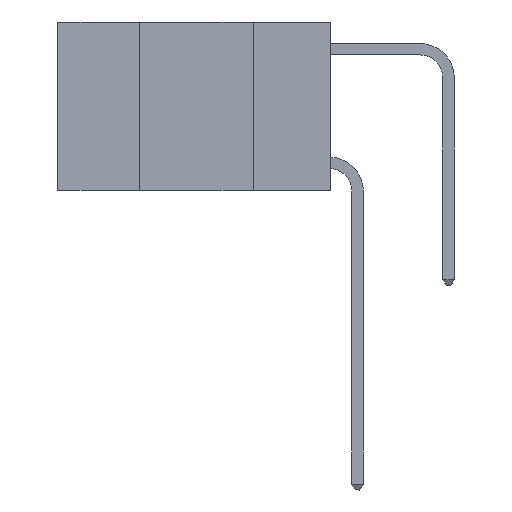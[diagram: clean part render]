
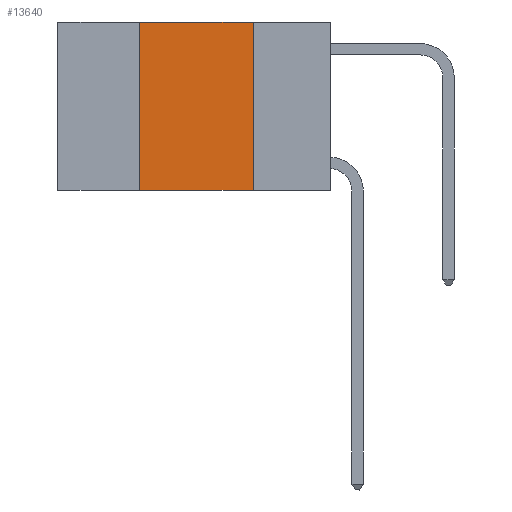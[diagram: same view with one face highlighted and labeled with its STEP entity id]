
A CAD part, left-side view. The second image highlights one B-rep face of the part: STEP entity #13640.
In plain terms, the highlighted planar face has unit normal (-1, 0, 0).
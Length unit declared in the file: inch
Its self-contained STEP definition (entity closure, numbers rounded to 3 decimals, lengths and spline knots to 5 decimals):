
#929 = VERTEX_POINT ( 'NONE', #13908 ) ;
#985 = ORIENTED_EDGE ( 'NONE', *, *, #4990, .F. ) ;
#1017 = VECTOR ( 'NONE', #14327, 39.37008 ) ;
#1131 = DIRECTION ( 'NONE',  ( 1., 0., 0. ) ) ;
#2269 = CARTESIAN_POINT ( 'NONE',  ( 0., 0.42, 0. ) ) ;
#4297 = EDGE_CURVE ( 'NONE', #929, #8619, #11769, .T. ) ;
#4489 = CARTESIAN_POINT ( 'NONE',  ( 0., 0.42, -0.37 ) ) ;
#4491 = CARTESIAN_POINT ( 'NONE',  ( 0., 0.17, -0.37 ) ) ;
#4765 = CARTESIAN_POINT ( 'NONE',  ( 0., 0.6, 0. ) ) ;
#4874 = VECTOR ( 'NONE', #16070, 39.37008 ) ;
#4990 = EDGE_CURVE ( 'NONE', #9619, #929, #16143, .T. ) ;
#5098 = ORIENTED_EDGE ( 'NONE', *, *, #14146, .F. ) ;
#5395 = VECTOR ( 'NONE', #12806, 39.37008 ) ;
#5797 = VECTOR ( 'NONE', #14953, 39.37008 ) ;
#6696 = FACE_OUTER_BOUND ( 'NONE', #9792, .T. ) ;
#8085 = CARTESIAN_POINT ( 'NONE',  ( 0., 0.42, 0. ) ) ;
#8619 = VERTEX_POINT ( 'NONE', #4491 ) ;
#8660 = CARTESIAN_POINT ( 'NONE',  ( 0., 0.17, 0. ) ) ;
#8819 = ORIENTED_EDGE ( 'NONE', *, *, #12000, .T. ) ;
#9490 = PLANE ( 'NONE',  #10551 ) ;
#9619 = VERTEX_POINT ( 'NONE', #8085 ) ;
#9792 = EDGE_LOOP ( 'NONE', ( #15484, #985, #5098, #8819 ) ) ;
#10551 = AXIS2_PLACEMENT_3D ( 'NONE', #17904, #1131, #10943 ) ;
#10943 = DIRECTION ( 'NONE',  ( 0., 0., -1. ) ) ;
#11422 = CARTESIAN_POINT ( 'NONE',  ( 0., 0.6, -0.37 ) ) ;
#11769 = LINE ( 'NONE', #8660, #1017 ) ;
#12000 = EDGE_CURVE ( 'NONE', #17609, #8619, #12933, .T. ) ;
#12806 = DIRECTION ( 'NONE',  ( 0., -1., 0. ) ) ;
#12933 = LINE ( 'NONE', #11422, #5395 ) ;
#13341 = LINE ( 'NONE', #2269, #5797 ) ;
#13640 = ADVANCED_FACE ( 'NONE', ( #6696 ), #9490, .F. ) ;
#13908 = CARTESIAN_POINT ( 'NONE',  ( 0., 0.17, 0. ) ) ;
#14146 = EDGE_CURVE ( 'NONE', #17609, #9619, #13341, .T. ) ;
#14327 = DIRECTION ( 'NONE',  ( 0., 0., -1. ) ) ;
#14953 = DIRECTION ( 'NONE',  ( 0., 0., 1. ) ) ;
#15484 = ORIENTED_EDGE ( 'NONE', *, *, #4297, .F. ) ;
#16070 = DIRECTION ( 'NONE',  ( 0., -1., 0. ) ) ;
#16143 = LINE ( 'NONE', #4765, #4874 ) ;
#17609 = VERTEX_POINT ( 'NONE', #4489 ) ;
#17904 = CARTESIAN_POINT ( 'NONE',  ( 0., 0.6, 0. ) ) ;
